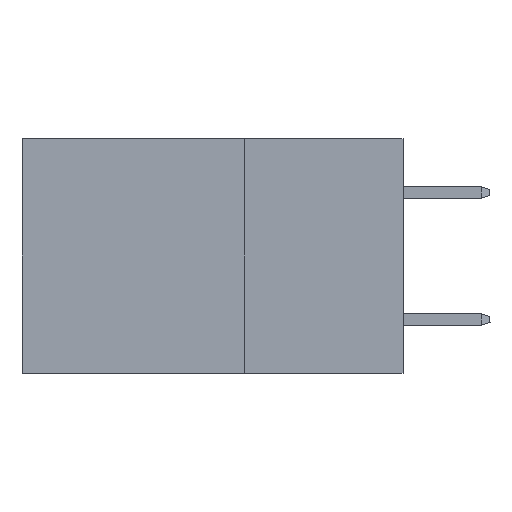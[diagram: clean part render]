
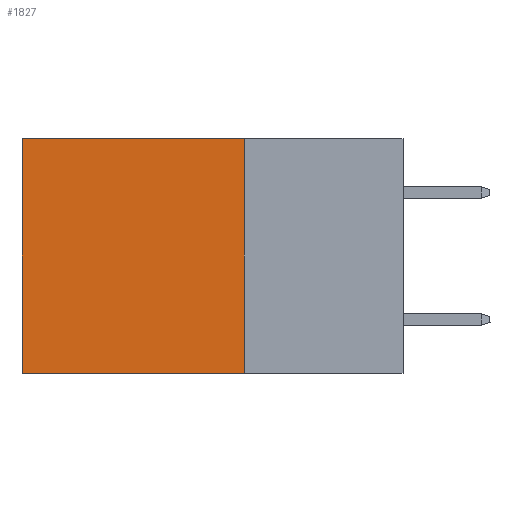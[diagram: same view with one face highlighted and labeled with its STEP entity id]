
A CAD part, left-side view. The second image highlights one B-rep face of the part: STEP entity #1827.
In plain terms, the highlighted planar face has unit normal (-1, 0, 0).
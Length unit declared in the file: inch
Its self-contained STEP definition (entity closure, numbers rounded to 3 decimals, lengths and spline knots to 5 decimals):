
#688 = LINE ( 'NONE', #6353, #2555 ) ;
#699 = EDGE_CURVE ( 'NONE', #9765, #9136, #688, .T. ) ;
#1827 = ADVANCED_FACE ( 'NONE', ( #11799 ), #26159, .F. ) ;
#1994 = VERTEX_POINT ( 'NONE', #12704 ) ;
#2555 = VECTOR ( 'NONE', #19023, 39.37008 ) ;
#5877 = CARTESIAN_POINT ( 'NONE',  ( 0.2875, 0.25, 0. ) ) ;
#5960 = LINE ( 'NONE', #26376, #15852 ) ;
#6353 = CARTESIAN_POINT ( 'NONE',  ( 0.2875, 0.25, 0. ) ) ;
#6752 = CARTESIAN_POINT ( 'NONE',  ( 0.2875, 0.25, 0. ) ) ;
#7567 = VECTOR ( 'NONE', #19405, 39.37008 ) ;
#8262 = EDGE_CURVE ( 'NONE', #9136, #1994, #5960, .T. ) ;
#9033 = LINE ( 'NONE', #15235, #7567 ) ;
#9136 = VERTEX_POINT ( 'NONE', #26416 ) ;
#9690 = AXIS2_PLACEMENT_3D ( 'NONE', #5877, #12186, #14069 ) ;
#9740 = VECTOR ( 'NONE', #13119, 39.37008 ) ;
#9765 = VERTEX_POINT ( 'NONE', #6752 ) ;
#10146 = CARTESIAN_POINT ( 'NONE',  ( 0.2875, 0.6, 0. ) ) ;
#10978 = CARTESIAN_POINT ( 'NONE',  ( 0.2875, 0.25, 0. ) ) ;
#11799 = FACE_OUTER_BOUND ( 'NONE', #13739, .T. ) ;
#12186 = DIRECTION ( 'NONE',  ( 1., 0., 0. ) ) ;
#12455 = VERTEX_POINT ( 'NONE', #10146 ) ;
#12704 = CARTESIAN_POINT ( 'NONE',  ( 0.2875, 0.6, -0.37 ) ) ;
#12816 = ORIENTED_EDGE ( 'NONE', *, *, #699, .F. ) ;
#13119 = DIRECTION ( 'NONE',  ( 0., 1., 0. ) ) ;
#13739 = EDGE_LOOP ( 'NONE', ( #20396, #23781, #12816, #19875 ) ) ;
#14069 = DIRECTION ( 'NONE',  ( 0., 0., -1. ) ) ;
#15235 = CARTESIAN_POINT ( 'NONE',  ( 0.2875, 0.6, 0. ) ) ;
#15852 = VECTOR ( 'NONE', #20611, 39.37008 ) ;
#17340 = LINE ( 'NONE', #10978, #9740 ) ;
#19023 = DIRECTION ( 'NONE',  ( 0., 0., -1. ) ) ;
#19405 = DIRECTION ( 'NONE',  ( 0., 0., -1. ) ) ;
#19415 = EDGE_CURVE ( 'NONE', #12455, #1994, #9033, .T. ) ;
#19875 = ORIENTED_EDGE ( 'NONE', *, *, #21811, .T. ) ;
#20396 = ORIENTED_EDGE ( 'NONE', *, *, #19415, .T. ) ;
#20611 = DIRECTION ( 'NONE',  ( 0., 1., 0. ) ) ;
#21811 = EDGE_CURVE ( 'NONE', #9765, #12455, #17340, .T. ) ;
#23781 = ORIENTED_EDGE ( 'NONE', *, *, #8262, .F. ) ;
#26159 = PLANE ( 'NONE',  #9690 ) ;
#26376 = CARTESIAN_POINT ( 'NONE',  ( 0.2875, 0.25, -0.37 ) ) ;
#26416 = CARTESIAN_POINT ( 'NONE',  ( 0.2875, 0.25, -0.37 ) ) ;
